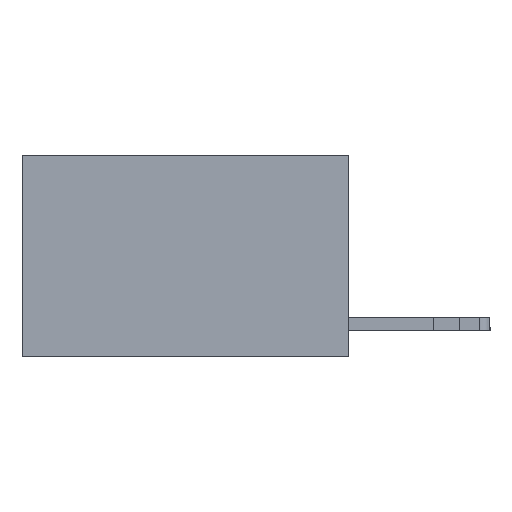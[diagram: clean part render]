
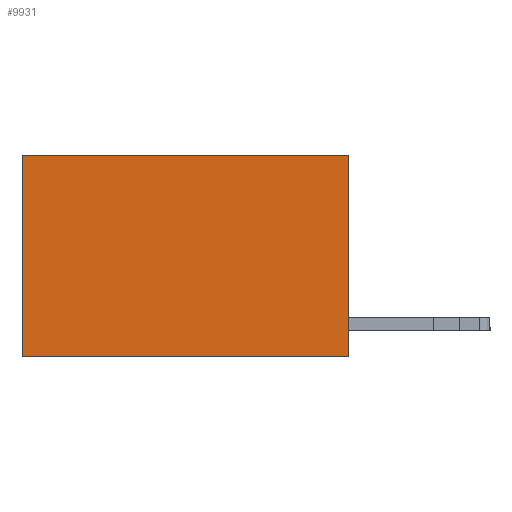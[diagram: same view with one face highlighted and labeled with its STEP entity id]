
A CAD part, left-side view. The second image highlights one B-rep face of the part: STEP entity #9931.
In plain terms, the highlighted planar face has unit normal (-1, 0, 0).
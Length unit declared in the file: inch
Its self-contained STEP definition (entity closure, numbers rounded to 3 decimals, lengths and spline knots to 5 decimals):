
#1504 = DIRECTION ( 'NONE',  ( 0., 0., -1. ) ) ;
#2236 = LINE ( 'NONE', #15403, #23951 ) ;
#3344 = VECTOR ( 'NONE', #9254, 39.37008 ) ;
#3522 = CARTESIAN_POINT ( 'NONE',  ( 0.2625, 0., 0. ) ) ;
#3959 = EDGE_CURVE ( 'NONE', #12560, #24119, #2236, .T. ) ;
#4813 = CARTESIAN_POINT ( 'NONE',  ( 0.2625, 0., 0. ) ) ;
#5126 = CARTESIAN_POINT ( 'NONE',  ( 0.2625, 0., -0.37 ) ) ;
#5283 = VECTOR ( 'NONE', #22350, 39.37008 ) ;
#7169 = FACE_OUTER_BOUND ( 'NONE', #18994, .T. ) ;
#7658 = PLANE ( 'NONE',  #23306 ) ;
#7983 = EDGE_CURVE ( 'NONE', #12560, #21791, #14708, .T. ) ;
#8023 = DIRECTION ( 'NONE',  ( 0., 0., -1. ) ) ;
#9254 = DIRECTION ( 'NONE',  ( 0., 1., 0. ) ) ;
#9749 = ORIENTED_EDGE ( 'NONE', *, *, #16378, .T. ) ;
#9931 = ADVANCED_FACE ( 'NONE', ( #7169 ), #7658, .F. ) ;
#11055 = CARTESIAN_POINT ( 'NONE',  ( 0.2625, 0.6, -0.37 ) ) ;
#11522 = EDGE_CURVE ( 'NONE', #24119, #20575, #19043, .T. ) ;
#12560 = VERTEX_POINT ( 'NONE', #14547 ) ;
#13014 = LINE ( 'NONE', #24422, #18901 ) ;
#13059 = CARTESIAN_POINT ( 'NONE',  ( 0.2625, 0.6, 0. ) ) ;
#13199 = ORIENTED_EDGE ( 'NONE', *, *, #3959, .F. ) ;
#14547 = CARTESIAN_POINT ( 'NONE',  ( 0.2625, 0., 0. ) ) ;
#14708 = LINE ( 'NONE', #4813, #5283 ) ;
#15124 = ORIENTED_EDGE ( 'NONE', *, *, #7983, .T. ) ;
#15403 = CARTESIAN_POINT ( 'NONE',  ( 0.2625, 0., 0. ) ) ;
#16378 = EDGE_CURVE ( 'NONE', #21791, #20575, #13014, .T. ) ;
#17039 = CARTESIAN_POINT ( 'NONE',  ( 0.2625, 0., -0.37 ) ) ;
#17165 = DIRECTION ( 'NONE',  ( 0., 0., -1. ) ) ;
#18901 = VECTOR ( 'NONE', #17165, 39.37008 ) ;
#18994 = EDGE_LOOP ( 'NONE', ( #9749, #23906, #13199, #15124 ) ) ;
#19043 = LINE ( 'NONE', #17039, #3344 ) ;
#20575 = VERTEX_POINT ( 'NONE', #11055 ) ;
#20812 = DIRECTION ( 'NONE',  ( 1., 0., 0. ) ) ;
#21791 = VERTEX_POINT ( 'NONE', #13059 ) ;
#22350 = DIRECTION ( 'NONE',  ( 0., 1., 0. ) ) ;
#23306 = AXIS2_PLACEMENT_3D ( 'NONE', #3522, #20812, #1504 ) ;
#23906 = ORIENTED_EDGE ( 'NONE', *, *, #11522, .F. ) ;
#23951 = VECTOR ( 'NONE', #8023, 39.37008 ) ;
#24119 = VERTEX_POINT ( 'NONE', #5126 ) ;
#24422 = CARTESIAN_POINT ( 'NONE',  ( 0.2625, 0.6, 0. ) ) ;
